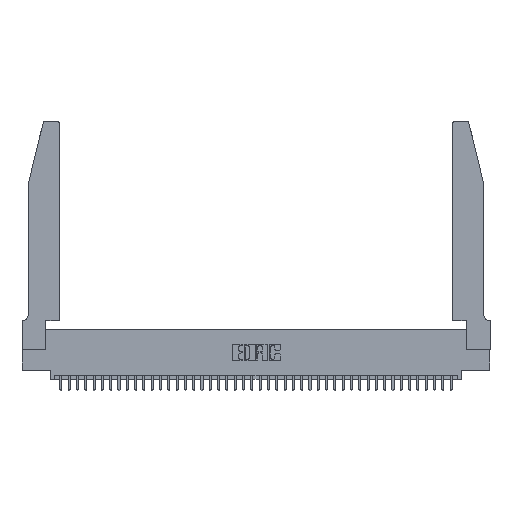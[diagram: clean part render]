
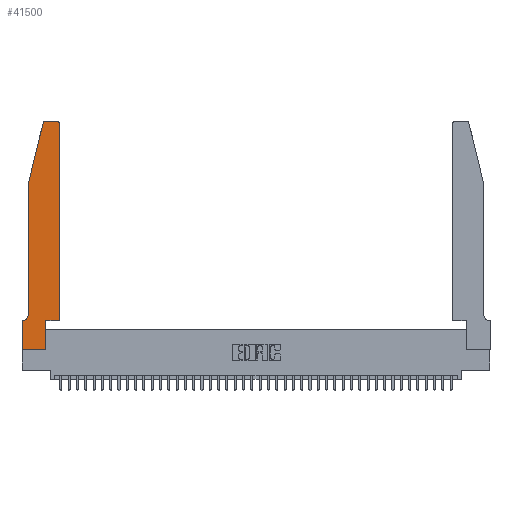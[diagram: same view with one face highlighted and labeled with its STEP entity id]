
A CAD part, top view. The second image highlights one B-rep face of the part: STEP entity #41500.
In plain terms, the highlighted planar face has unit normal (0, 0, 1).
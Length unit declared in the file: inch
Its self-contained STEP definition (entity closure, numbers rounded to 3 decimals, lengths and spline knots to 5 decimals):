
#82 = VERTEX_POINT ( 'NONE', #9266 ) ;
#772 = DIRECTION ( 'NONE',  ( -1., 0., 0. ) ) ;
#901 = VERTEX_POINT ( 'NONE', #40727 ) ;
#961 = DIRECTION ( 'NONE',  ( 0., 1., 0. ) ) ;
#1387 = DIRECTION ( 'NONE',  ( -1., 0., 0. ) ) ;
#1551 = CARTESIAN_POINT ( 'NONE',  ( 0.0755, 0.42, 0.37 ) ) ;
#1584 = DIRECTION ( 'NONE',  ( 1., 0., 0. ) ) ;
#1650 = ORIENTED_EDGE ( 'NONE', *, *, #4823, .T. ) ;
#2226 = CARTESIAN_POINT ( 'NONE',  ( 0., 0.35, 0.37 ) ) ;
#2633 = VECTOR ( 'NONE', #15044, 39.37008 ) ;
#2807 = CARTESIAN_POINT ( 'NONE',  ( 0., 0., 0.37 ) ) ;
#3257 = LINE ( 'NONE', #24381, #19397 ) ;
#3346 = ORIENTED_EDGE ( 'NONE', *, *, #11905, .T. ) ;
#3746 = DIRECTION ( 'NONE',  ( 0., -1., 0. ) ) ;
#3978 = CIRCLE ( 'NONE', #35539, 0.07 ) ;
#4372 = CARTESIAN_POINT ( 'NONE',  ( 0.284, 2.72, 0.37 ) ) ;
#4639 = LINE ( 'NONE', #5276, #2633 ) ;
#4725 = EDGE_CURVE ( 'NONE', #24120, #82, #3978, .T. ) ;
#4823 = EDGE_CURVE ( 'NONE', #36683, #23820, #9024, .T. ) ;
#4990 = VECTOR ( 'NONE', #961, 39.37008 ) ;
#5276 = CARTESIAN_POINT ( 'NONE',  ( 0., 0., 0.37 ) ) ;
#5638 = LINE ( 'NONE', #40835, #31423 ) ;
#6071 = CIRCLE ( 'NONE', #14879, 0.03 ) ;
#7538 = CARTESIAN_POINT ( 'NONE',  ( 0.284, 2.75, 0.37 ) ) ;
#7951 = EDGE_CURVE ( 'NONE', #23820, #23627, #3257, .T. ) ;
#8668 = ORIENTED_EDGE ( 'NONE', *, *, #4725, .T. ) ;
#9024 = LINE ( 'NONE', #39625, #4990 ) ;
#9189 = EDGE_CURVE ( 'NONE', #23627, #37012, #5638, .T. ) ;
#9266 = CARTESIAN_POINT ( 'NONE',  ( 0.0055, 0.35, 0.37 ) ) ;
#10514 = CARTESIAN_POINT ( 'NONE',  ( 0.4205, 2.75, 0.37 ) ) ;
#11905 = EDGE_CURVE ( 'NONE', #17910, #36683, #4639, .T. ) ;
#12032 = CARTESIAN_POINT ( 'NONE',  ( 0., 0., 0.37 ) ) ;
#12146 = LINE ( 'NONE', #16473, #19665 ) ;
#12268 = ORIENTED_EDGE ( 'NONE', *, *, #37274, .T. ) ;
#13796 = EDGE_CURVE ( 'NONE', #82, #15511, #12146, .T. ) ;
#13855 = VERTEX_POINT ( 'NONE', #7538 ) ;
#14111 = LINE ( 'NONE', #2807, #28754 ) ;
#14641 = AXIS2_PLACEMENT_3D ( 'NONE', #40243, #40663, #1584 ) ;
#14879 = AXIS2_PLACEMENT_3D ( 'NONE', #4372, #20563, #26950 ) ;
#15044 = DIRECTION ( 'NONE',  ( 1., 0., 0. ) ) ;
#15113 = LINE ( 'NONE', #30602, #36290 ) ;
#15312 = EDGE_CURVE ( 'NONE', #16907, #13855, #15113, .T. ) ;
#15511 = VERTEX_POINT ( 'NONE', #2226 ) ;
#15756 = CARTESIAN_POINT ( 'NONE',  ( 0., 0.35, 0.37 ) ) ;
#15807 = DIRECTION ( 'NONE',  ( 0., -1., 0. ) ) ;
#16473 = CARTESIAN_POINT ( 'NONE',  ( 0.0755, 0.35, 0.37 ) ) ;
#16907 = VERTEX_POINT ( 'NONE', #10514 ) ;
#17130 = AXIS2_PLACEMENT_3D ( 'NONE', #15756, #38301, #28433 ) ;
#17910 = VERTEX_POINT ( 'NONE', #12032 ) ;
#17998 = CARTESIAN_POINT ( 'NONE',  ( 0.4505, 2.72, 0.37 ) ) ;
#18085 = CARTESIAN_POINT ( 'NONE',  ( 0.4505, 0.35, 0.37 ) ) ;
#19219 = CARTESIAN_POINT ( 'NONE',  ( 0.2865, 0.35, 0.37 ) ) ;
#19340 = ORIENTED_EDGE ( 'NONE', *, *, #41029, .T. ) ;
#19397 = VECTOR ( 'NONE', #40356, 39.37008 ) ;
#19665 = VECTOR ( 'NONE', #772, 39.37008 ) ;
#20563 = DIRECTION ( 'NONE',  ( 0., 0., 1. ) ) ;
#21695 = ORIENTED_EDGE ( 'NONE', *, *, #25310, .T. ) ;
#22552 = EDGE_CURVE ( 'NONE', #15511, #17910, #14111, .T. ) ;
#23521 = CARTESIAN_POINT ( 'NONE',  ( 0.0055, 0.42, 0.37 ) ) ;
#23625 = EDGE_CURVE ( 'NONE', #37012, #16907, #28125, .T. ) ;
#23627 = VERTEX_POINT ( 'NONE', #18085 ) ;
#23820 = VERTEX_POINT ( 'NONE', #19219 ) ;
#24120 = VERTEX_POINT ( 'NONE', #1551 ) ;
#24381 = CARTESIAN_POINT ( 'NONE',  ( 0.4505, 0.35, 0.37 ) ) ;
#25310 = EDGE_CURVE ( 'NONE', #13855, #40548, #6071, .T. ) ;
#25453 = CARTESIAN_POINT ( 'NONE',  ( 0.0755, 2., 0.37 ) ) ;
#26338 = CARTESIAN_POINT ( 'NONE',  ( 0.2865, 0., 0.37 ) ) ;
#26379 = LINE ( 'NONE', #25453, #34485 ) ;
#26416 = ORIENTED_EDGE ( 'NONE', *, *, #22552, .T. ) ;
#26629 = LINE ( 'NONE', #33099, #27126 ) ;
#26950 = DIRECTION ( 'NONE',  ( 1., 0., 0. ) ) ;
#27126 = VECTOR ( 'NONE', #3746, 39.37008 ) ;
#28125 = CIRCLE ( 'NONE', #14641, 0.03 ) ;
#28433 = DIRECTION ( 'NONE',  ( 1., 0., 0. ) ) ;
#28571 = DIRECTION ( 'NONE',  ( -0.239, -0.971, 0. ) ) ;
#28754 = VECTOR ( 'NONE', #15807, 39.37008 ) ;
#29814 = ORIENTED_EDGE ( 'NONE', *, *, #7951, .T. ) ;
#30602 = CARTESIAN_POINT ( 'NONE',  ( 0.2605, 2.75, 0.37 ) ) ;
#31423 = VECTOR ( 'NONE', #40407, 39.37008 ) ;
#32871 = DIRECTION ( 'NONE',  ( 0., 0., -1. ) ) ;
#33071 = ORIENTED_EDGE ( 'NONE', *, *, #13796, .T. ) ;
#33099 = CARTESIAN_POINT ( 'NONE',  ( 0.0755, 2., 0.37 ) ) ;
#34485 = VECTOR ( 'NONE', #28571, 39.37008 ) ;
#34994 = ORIENTED_EDGE ( 'NONE', *, *, #9189, .T. ) ;
#35539 = AXIS2_PLACEMENT_3D ( 'NONE', #23521, #32871, #36096 ) ;
#36096 = DIRECTION ( 'NONE',  ( -1., 0., 0. ) ) ;
#36290 = VECTOR ( 'NONE', #1387, 39.37008 ) ;
#36585 = EDGE_LOOP ( 'NONE', ( #38229, #21695, #12268, #19340, #8668, #33071, #26416, #3346, #1650, #29814, #34994, #38705 ) ) ;
#36683 = VERTEX_POINT ( 'NONE', #26338 ) ;
#37012 = VERTEX_POINT ( 'NONE', #17998 ) ;
#37274 = EDGE_CURVE ( 'NONE', #40548, #901, #26379, .T. ) ;
#38166 = PLANE ( 'NONE',  #17130 ) ;
#38229 = ORIENTED_EDGE ( 'NONE', *, *, #15312, .T. ) ;
#38301 = DIRECTION ( 'NONE',  ( 0., 0., 1. ) ) ;
#38705 = ORIENTED_EDGE ( 'NONE', *, *, #23625, .T. ) ;
#39625 = CARTESIAN_POINT ( 'NONE',  ( 0.2865, 0.35, 0.37 ) ) ;
#40243 = CARTESIAN_POINT ( 'NONE',  ( 0.4205, 2.72, 0.37 ) ) ;
#40356 = DIRECTION ( 'NONE',  ( 1., 0., 0. ) ) ;
#40407 = DIRECTION ( 'NONE',  ( 0., 1., 0. ) ) ;
#40548 = VERTEX_POINT ( 'NONE', #41745 ) ;
#40663 = DIRECTION ( 'NONE',  ( 0., 0., 1. ) ) ;
#40727 = CARTESIAN_POINT ( 'NONE',  ( 0.0755, 2., 0.37 ) ) ;
#40732 = FACE_OUTER_BOUND ( 'NONE', #36585, .T. ) ;
#40835 = CARTESIAN_POINT ( 'NONE',  ( 0.4505, 0.35, 0.37 ) ) ;
#41029 = EDGE_CURVE ( 'NONE', #901, #24120, #26629, .T. ) ;
#41500 = ADVANCED_FACE ( 'NONE', ( #40732 ), #38166, .T. ) ;
#41745 = CARTESIAN_POINT ( 'NONE',  ( 0.25487, 2.72718, 0.37 ) ) ;
